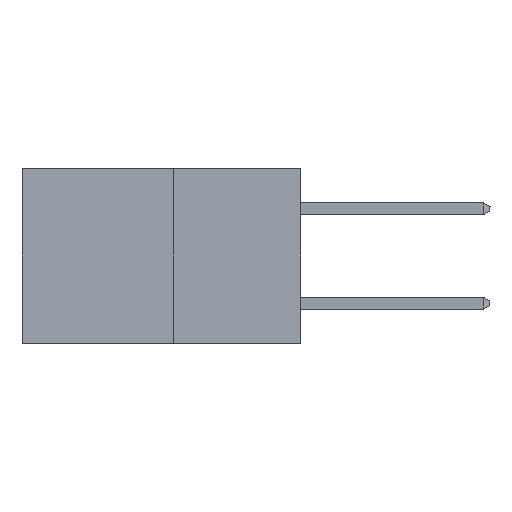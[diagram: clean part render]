
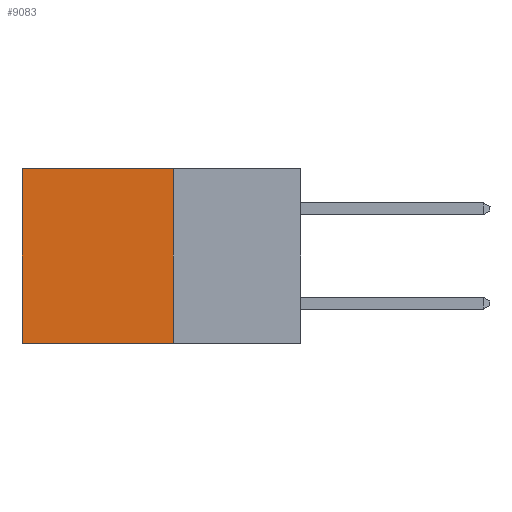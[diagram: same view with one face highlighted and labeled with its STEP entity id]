
A CAD part, left-side view. The second image highlights one B-rep face of the part: STEP entity #9083.
In plain terms, the highlighted planar face has unit normal (-1, 0, 0).
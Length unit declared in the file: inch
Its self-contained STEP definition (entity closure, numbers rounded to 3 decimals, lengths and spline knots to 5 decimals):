
#399 = LINE ( 'NONE', #510, #14999 ) ;
#496 = EDGE_CURVE ( 'NONE', #8493, #12904, #399, .T. ) ;
#510 = CARTESIAN_POINT ( 'NONE',  ( 0.277, 0.59, -0.37 ) ) ;
#706 = CARTESIAN_POINT ( 'NONE',  ( 0.277, 0.59, -0.37 ) ) ;
#1626 = CARTESIAN_POINT ( 'NONE',  ( 0.277, 0.27, -0.37 ) ) ;
#2495 = VECTOR ( 'NONE', #13204, 39.37008 ) ;
#3058 = VERTEX_POINT ( 'NONE', #6141 ) ;
#4373 = FACE_OUTER_BOUND ( 'NONE', #10285, .T. ) ;
#4759 = CARTESIAN_POINT ( 'NONE',  ( 0.277, 0.27, 0. ) ) ;
#4966 = CARTESIAN_POINT ( 'NONE',  ( 0.277, 0.27, -0.37 ) ) ;
#6141 = CARTESIAN_POINT ( 'NONE',  ( 0.277, 0.27, 0. ) ) ;
#6290 = DIRECTION ( 'NONE',  ( 0., 1., 0. ) ) ;
#6317 = LINE ( 'NONE', #4759, #2495 ) ;
#6408 = DIRECTION ( 'NONE',  ( 0., 0., -1. ) ) ;
#6488 = ORIENTED_EDGE ( 'NONE', *, *, #17850, .T. ) ;
#8066 = DIRECTION ( 'NONE',  ( 0., 0., -1. ) ) ;
#8493 = VERTEX_POINT ( 'NONE', #12155 ) ;
#9083 = ADVANCED_FACE ( 'NONE', ( #4373 ), #9198, .F. ) ;
#9198 = PLANE ( 'NONE',  #9662 ) ;
#9599 = EDGE_CURVE ( 'NONE', #3058, #10000, #14043, .T. ) ;
#9662 = AXIS2_PLACEMENT_3D ( 'NONE', #4966, #14784, #6408 ) ;
#10000 = VERTEX_POINT ( 'NONE', #1626 ) ;
#10285 = EDGE_LOOP ( 'NONE', ( #17089, #13081, #14101, #6488 ) ) ;
#11168 = EDGE_CURVE ( 'NONE', #10000, #12904, #13355, .T. ) ;
#11870 = DIRECTION ( 'NONE',  ( 0., 0., -1. ) ) ;
#12155 = CARTESIAN_POINT ( 'NONE',  ( 0.277, 0.59, 0. ) ) ;
#12904 = VERTEX_POINT ( 'NONE', #706 ) ;
#13081 = ORIENTED_EDGE ( 'NONE', *, *, #11168, .F. ) ;
#13204 = DIRECTION ( 'NONE',  ( 0., 1., 0. ) ) ;
#13355 = LINE ( 'NONE', #14665, #16558 ) ;
#14043 = LINE ( 'NONE', #17345, #14904 ) ;
#14101 = ORIENTED_EDGE ( 'NONE', *, *, #9599, .F. ) ;
#14665 = CARTESIAN_POINT ( 'NONE',  ( 0.277, 0.27, -0.37 ) ) ;
#14784 = DIRECTION ( 'NONE',  ( 1., 0., 0. ) ) ;
#14904 = VECTOR ( 'NONE', #11870, 39.37008 ) ;
#14999 = VECTOR ( 'NONE', #8066, 39.37008 ) ;
#16558 = VECTOR ( 'NONE', #6290, 39.37008 ) ;
#17089 = ORIENTED_EDGE ( 'NONE', *, *, #496, .T. ) ;
#17345 = CARTESIAN_POINT ( 'NONE',  ( 0.277, 0.27, -0.37 ) ) ;
#17850 = EDGE_CURVE ( 'NONE', #3058, #8493, #6317, .T. ) ;
